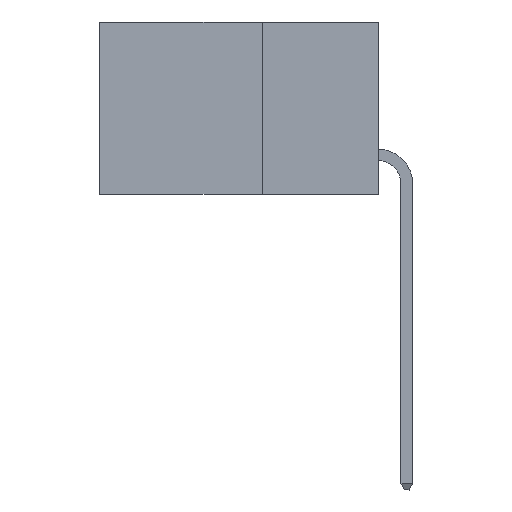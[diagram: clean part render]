
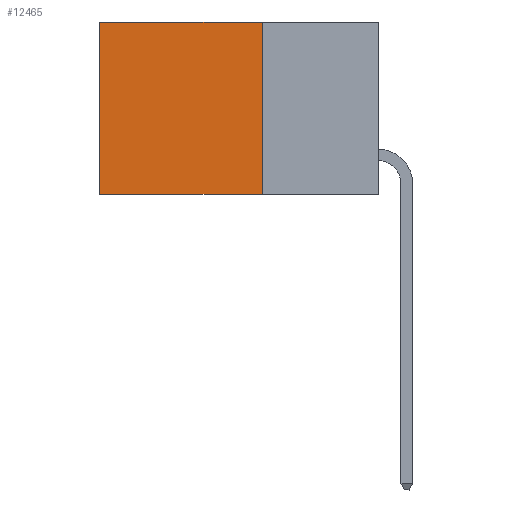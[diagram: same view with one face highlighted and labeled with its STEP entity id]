
A CAD part, left-side view. The second image highlights one B-rep face of the part: STEP entity #12465.
In plain terms, the highlighted planar face has unit normal (-1, 0, 0).
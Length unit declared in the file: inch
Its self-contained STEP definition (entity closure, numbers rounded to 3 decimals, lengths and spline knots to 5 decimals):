
#388 = VECTOR ( 'NONE', #9307, 39.37008 ) ;
#564 = CARTESIAN_POINT ( 'NONE',  ( 0.2615, 0.25, 0. ) ) ;
#1138 = VERTEX_POINT ( 'NONE', #8335 ) ;
#2068 = DIRECTION ( 'NONE',  ( 0., 1., 0. ) ) ;
#2211 = EDGE_CURVE ( 'NONE', #2802, #1138, #10326, .T. ) ;
#2772 = CARTESIAN_POINT ( 'NONE',  ( 0.2615, 0.6, 0. ) ) ;
#2802 = VERTEX_POINT ( 'NONE', #7256 ) ;
#3660 = CARTESIAN_POINT ( 'NONE',  ( 0.2615, 0.6, -0.37 ) ) ;
#3665 = CARTESIAN_POINT ( 'NONE',  ( 0.2615, 0.25, -0.37 ) ) ;
#3792 = VECTOR ( 'NONE', #4992, 39.37008 ) ;
#4782 = EDGE_CURVE ( 'NONE', #12593, #2802, #12303, .T. ) ;
#4795 = DIRECTION ( 'NONE',  ( 0., 0., -1. ) ) ;
#4992 = DIRECTION ( 'NONE',  ( 0., 0., -1. ) ) ;
#5224 = CARTESIAN_POINT ( 'NONE',  ( 0.2615, 0.25, -0.37 ) ) ;
#6225 = EDGE_LOOP ( 'NONE', ( #7479, #10604, #12660, #10512 ) ) ;
#6237 = EDGE_CURVE ( 'NONE', #12593, #6762, #9427, .T. ) ;
#6762 = VERTEX_POINT ( 'NONE', #2772 ) ;
#7256 = CARTESIAN_POINT ( 'NONE',  ( 0.2615, 0.25, -0.37 ) ) ;
#7304 = VECTOR ( 'NONE', #8882, 39.37008 ) ;
#7479 = ORIENTED_EDGE ( 'NONE', *, *, #11251, .T. ) ;
#7752 = LINE ( 'NONE', #3660, #7304 ) ;
#7755 = DIRECTION ( 'NONE',  ( 1., 0., 0. ) ) ;
#7822 = PLANE ( 'NONE',  #9866 ) ;
#8335 = CARTESIAN_POINT ( 'NONE',  ( 0.2615, 0.6, -0.37 ) ) ;
#8882 = DIRECTION ( 'NONE',  ( 0., 0., -1. ) ) ;
#9277 = CARTESIAN_POINT ( 'NONE',  ( 0.2615, 0.25, -0.37 ) ) ;
#9307 = DIRECTION ( 'NONE',  ( 0., 1., 0. ) ) ;
#9427 = LINE ( 'NONE', #12461, #11695 ) ;
#9866 = AXIS2_PLACEMENT_3D ( 'NONE', #3665, #7755, #4795 ) ;
#10326 = LINE ( 'NONE', #5224, #388 ) ;
#10512 = ORIENTED_EDGE ( 'NONE', *, *, #6237, .T. ) ;
#10604 = ORIENTED_EDGE ( 'NONE', *, *, #2211, .F. ) ;
#11251 = EDGE_CURVE ( 'NONE', #6762, #1138, #7752, .T. ) ;
#11695 = VECTOR ( 'NONE', #2068, 39.37008 ) ;
#11913 = FACE_OUTER_BOUND ( 'NONE', #6225, .T. ) ;
#12303 = LINE ( 'NONE', #9277, #3792 ) ;
#12461 = CARTESIAN_POINT ( 'NONE',  ( 0.2615, 0.25, 0. ) ) ;
#12465 = ADVANCED_FACE ( 'NONE', ( #11913 ), #7822, .F. ) ;
#12593 = VERTEX_POINT ( 'NONE', #564 ) ;
#12660 = ORIENTED_EDGE ( 'NONE', *, *, #4782, .F. ) ;
